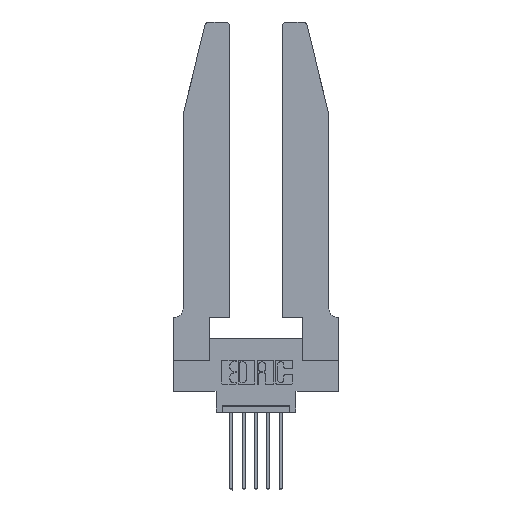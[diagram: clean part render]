
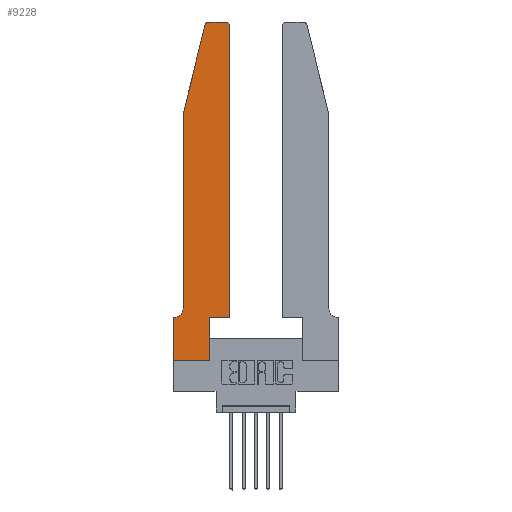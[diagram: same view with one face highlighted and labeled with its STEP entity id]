
A CAD part, top view. The second image highlights one B-rep face of the part: STEP entity #9228.
In plain terms, the highlighted planar face has unit normal (0, 0, 1).
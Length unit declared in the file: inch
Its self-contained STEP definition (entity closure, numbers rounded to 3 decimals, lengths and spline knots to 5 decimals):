
#105 = ORIENTED_EDGE ( 'NONE', *, *, #11975, .T. ) ;
#161 = EDGE_CURVE ( 'NONE', #1682, #6223, #2447, .T. ) ;
#269 = VERTEX_POINT ( 'NONE', #4859 ) ;
#461 = ORIENTED_EDGE ( 'NONE', *, *, #12179, .T. ) ;
#622 = VECTOR ( 'NONE', #3390, 39.37008 ) ;
#702 = LINE ( 'NONE', #5400, #10096 ) ;
#885 = EDGE_CURVE ( 'NONE', #8715, #6215, #11999, .T. ) ;
#924 = VECTOR ( 'NONE', #2334, 39.37008 ) ;
#987 = CIRCLE ( 'NONE', #9888, 0.03 ) ;
#1202 = CARTESIAN_POINT ( 'NONE',  ( 0.4205, 2.72, 0.37 ) ) ;
#1447 = LINE ( 'NONE', #7444, #6389 ) ;
#1499 = CARTESIAN_POINT ( 'NONE',  ( 0., 0.35, 0.37 ) ) ;
#1571 = CARTESIAN_POINT ( 'NONE',  ( 0.0755, 2., 0.37 ) ) ;
#1595 = DIRECTION ( 'NONE',  ( 1., 0., 0. ) ) ;
#1682 = VERTEX_POINT ( 'NONE', #10745 ) ;
#1874 = CARTESIAN_POINT ( 'NONE',  ( 0.284, 2.72, 0.37 ) ) ;
#1969 = DIRECTION ( 'NONE',  ( 0., 0., 1. ) ) ;
#1986 = CARTESIAN_POINT ( 'NONE',  ( 0.0755, 0.35, 0.37 ) ) ;
#2310 = CARTESIAN_POINT ( 'NONE',  ( 0.0755, 2., 0.37 ) ) ;
#2334 = DIRECTION ( 'NONE',  ( -1., 0., 0. ) ) ;
#2447 = LINE ( 'NONE', #6353, #7704 ) ;
#2533 = CARTESIAN_POINT ( 'NONE',  ( 0.0055, 0.35, 0.37 ) ) ;
#2634 = DIRECTION ( 'NONE',  ( 0., -1., 0. ) ) ;
#2877 = ORIENTED_EDGE ( 'NONE', *, *, #13647, .T. ) ;
#2949 = AXIS2_PLACEMENT_3D ( 'NONE', #8289, #6135, #4041 ) ;
#3390 = DIRECTION ( 'NONE',  ( 0., 1., 0. ) ) ;
#3549 = ORIENTED_EDGE ( 'NONE', *, *, #161, .T. ) ;
#3624 = DIRECTION ( 'NONE',  ( 0., 0., 1. ) ) ;
#3709 = EDGE_CURVE ( 'NONE', #7758, #8529, #13081, .T. ) ;
#4041 = DIRECTION ( 'NONE',  ( -1., 0., 0. ) ) ;
#4324 = DIRECTION ( 'NONE',  ( 1., 0., 0. ) ) ;
#4859 = CARTESIAN_POINT ( 'NONE',  ( 0., 0.35, 0.37 ) ) ;
#4993 = CARTESIAN_POINT ( 'NONE',  ( 0.284, 2.75, 0.37 ) ) ;
#5352 = EDGE_CURVE ( 'NONE', #6215, #12190, #9559, .T. ) ;
#5400 = CARTESIAN_POINT ( 'NONE',  ( 0.4505, 0.35, 0.37 ) ) ;
#5783 = ORIENTED_EDGE ( 'NONE', *, *, #8165, .T. ) ;
#5798 = VECTOR ( 'NONE', #13615, 39.37008 ) ;
#5804 = AXIS2_PLACEMENT_3D ( 'NONE', #1499, #3624, #1595 ) ;
#5807 = EDGE_CURVE ( 'NONE', #10396, #6227, #11881, .T. ) ;
#6047 = EDGE_CURVE ( 'NONE', #6227, #7758, #13179, .T. ) ;
#6135 = DIRECTION ( 'NONE',  ( 0., 0., -1. ) ) ;
#6215 = VERTEX_POINT ( 'NONE', #10165 ) ;
#6223 = VERTEX_POINT ( 'NONE', #7120 ) ;
#6227 = VERTEX_POINT ( 'NONE', #8183 ) ;
#6315 = DIRECTION ( 'NONE',  ( 1., 0., 0. ) ) ;
#6353 = CARTESIAN_POINT ( 'NONE',  ( 0.2865, 0.35, 0.37 ) ) ;
#6389 = VECTOR ( 'NONE', #4324, 39.37008 ) ;
#6847 = FACE_OUTER_BOUND ( 'NONE', #8066, .T. ) ;
#7120 = CARTESIAN_POINT ( 'NONE',  ( 0.2865, 0.35, 0.37 ) ) ;
#7247 = DIRECTION ( 'NONE',  ( 1., 0., 0. ) ) ;
#7444 = CARTESIAN_POINT ( 'NONE',  ( 0., 0., 0.37 ) ) ;
#7704 = VECTOR ( 'NONE', #13093, 39.37008 ) ;
#7758 = VERTEX_POINT ( 'NONE', #10040 ) ;
#7948 = LINE ( 'NONE', #1986, #5798 ) ;
#8066 = EDGE_LOOP ( 'NONE', ( #8167, #2877, #9946, #10854, #11364, #461, #12791, #5783, #3549, #105, #9736, #9574 ) ) ;
#8086 = EDGE_CURVE ( 'NONE', #269, #12529, #12314, .T. ) ;
#8165 = EDGE_CURVE ( 'NONE', #12529, #1682, #1447, .T. ) ;
#8167 = ORIENTED_EDGE ( 'NONE', *, *, #9018, .T. ) ;
#8183 = CARTESIAN_POINT ( 'NONE',  ( 0.0755, 2., 0.37 ) ) ;
#8289 = CARTESIAN_POINT ( 'NONE',  ( 0.0055, 0.42, 0.37 ) ) ;
#8399 = VECTOR ( 'NONE', #8504, 39.37008 ) ;
#8504 = DIRECTION ( 'NONE',  ( -0.239, -0.971, 0. ) ) ;
#8529 = VERTEX_POINT ( 'NONE', #2533 ) ;
#8615 = CARTESIAN_POINT ( 'NONE',  ( 0.2605, 2.75, 0.37 ) ) ;
#8715 = VERTEX_POINT ( 'NONE', #13204 ) ;
#8719 = CARTESIAN_POINT ( 'NONE',  ( 0., 0., 0.37 ) ) ;
#8899 = CARTESIAN_POINT ( 'NONE',  ( 0.25487, 2.72718, 0.37 ) ) ;
#9018 = EDGE_CURVE ( 'NONE', #12190, #9548, #9305, .T. ) ;
#9189 = AXIS2_PLACEMENT_3D ( 'NONE', #1202, #9522, #6315 ) ;
#9228 = ADVANCED_FACE ( 'NONE', ( #6847 ), #9860, .T. ) ;
#9305 = LINE ( 'NONE', #8615, #924 ) ;
#9415 = CARTESIAN_POINT ( 'NONE',  ( 0., 0., 0.37 ) ) ;
#9522 = DIRECTION ( 'NONE',  ( 0., 0., 1. ) ) ;
#9544 = VECTOR ( 'NONE', #2634, 39.37008 ) ;
#9548 = VERTEX_POINT ( 'NONE', #4993 ) ;
#9559 = CIRCLE ( 'NONE', #9189, 0.03 ) ;
#9574 = ORIENTED_EDGE ( 'NONE', *, *, #5352, .T. ) ;
#9736 = ORIENTED_EDGE ( 'NONE', *, *, #885, .T. ) ;
#9860 = PLANE ( 'NONE',  #5804 ) ;
#9888 = AXIS2_PLACEMENT_3D ( 'NONE', #1874, #1969, #7247 ) ;
#9946 = ORIENTED_EDGE ( 'NONE', *, *, #5807, .T. ) ;
#10040 = CARTESIAN_POINT ( 'NONE',  ( 0.0755, 0.42, 0.37 ) ) ;
#10096 = VECTOR ( 'NONE', #11985, 39.37008 ) ;
#10165 = CARTESIAN_POINT ( 'NONE',  ( 0.4505, 2.72, 0.37 ) ) ;
#10170 = VECTOR ( 'NONE', #13560, 39.37008 ) ;
#10396 = VERTEX_POINT ( 'NONE', #8899 ) ;
#10745 = CARTESIAN_POINT ( 'NONE',  ( 0.2865, 0., 0.37 ) ) ;
#10854 = ORIENTED_EDGE ( 'NONE', *, *, #6047, .T. ) ;
#11364 = ORIENTED_EDGE ( 'NONE', *, *, #3709, .T. ) ;
#11417 = CARTESIAN_POINT ( 'NONE',  ( 0.4205, 2.75, 0.37 ) ) ;
#11881 = LINE ( 'NONE', #2310, #8399 ) ;
#11912 = CARTESIAN_POINT ( 'NONE',  ( 0.4505, 0.35, 0.37 ) ) ;
#11975 = EDGE_CURVE ( 'NONE', #6223, #8715, #702, .T. ) ;
#11985 = DIRECTION ( 'NONE',  ( 1., 0., 0. ) ) ;
#11999 = LINE ( 'NONE', #11912, #622 ) ;
#12179 = EDGE_CURVE ( 'NONE', #8529, #269, #7948, .T. ) ;
#12190 = VERTEX_POINT ( 'NONE', #11417 ) ;
#12314 = LINE ( 'NONE', #9415, #10170 ) ;
#12529 = VERTEX_POINT ( 'NONE', #8719 ) ;
#12791 = ORIENTED_EDGE ( 'NONE', *, *, #8086, .T. ) ;
#13081 = CIRCLE ( 'NONE', #2949, 0.07 ) ;
#13093 = DIRECTION ( 'NONE',  ( 0., 1., 0. ) ) ;
#13179 = LINE ( 'NONE', #1571, #9544 ) ;
#13204 = CARTESIAN_POINT ( 'NONE',  ( 0.4505, 0.35, 0.37 ) ) ;
#13560 = DIRECTION ( 'NONE',  ( 0., -1., 0. ) ) ;
#13615 = DIRECTION ( 'NONE',  ( -1., 0., 0. ) ) ;
#13647 = EDGE_CURVE ( 'NONE', #9548, #10396, #987, .T. ) ;
